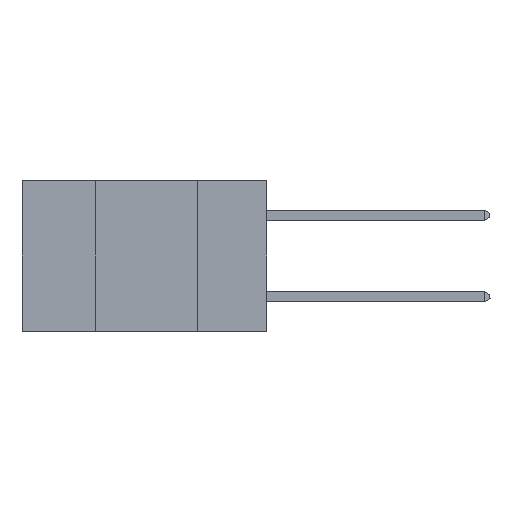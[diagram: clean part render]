
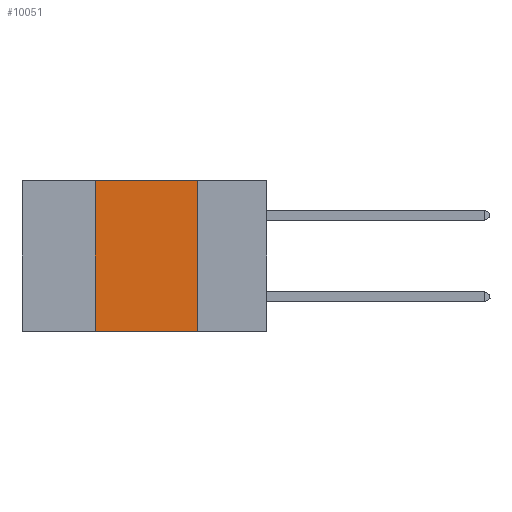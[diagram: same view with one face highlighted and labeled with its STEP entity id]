
A CAD part, left-side view. The second image highlights one B-rep face of the part: STEP entity #10051.
In plain terms, the highlighted planar face has unit normal (-1, 0, 0).
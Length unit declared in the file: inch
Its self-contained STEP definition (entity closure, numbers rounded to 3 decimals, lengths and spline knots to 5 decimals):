
#732 = CARTESIAN_POINT ( 'NONE',  ( 0., 0.17, 0. ) ) ;
#1130 = DIRECTION ( 'NONE',  ( 0., -1., 0. ) ) ;
#2882 = LINE ( 'NONE', #7137, #13762 ) ;
#3094 = ORIENTED_EDGE ( 'NONE', *, *, #14947, .F. ) ;
#3384 = EDGE_LOOP ( 'NONE', ( #3094, #11503, #5158, #14733 ) ) ;
#3385 = CARTESIAN_POINT ( 'NONE',  ( 0., 0.6, -0.37 ) ) ;
#3785 = VERTEX_POINT ( 'NONE', #13073 ) ;
#4126 = EDGE_CURVE ( 'NONE', #13854, #11864, #10080, .T. ) ;
#4193 = LINE ( 'NONE', #732, #5136 ) ;
#4670 = PLANE ( 'NONE',  #7033 ) ;
#5136 = VECTOR ( 'NONE', #6911, 39.37008 ) ;
#5158 = ORIENTED_EDGE ( 'NONE', *, *, #7703, .F. ) ;
#6596 = CARTESIAN_POINT ( 'NONE',  ( 0., 0.42, 0. ) ) ;
#6760 = VERTEX_POINT ( 'NONE', #15274 ) ;
#6911 = DIRECTION ( 'NONE',  ( 0., 0., -1. ) ) ;
#7033 = AXIS2_PLACEMENT_3D ( 'NONE', #14284, #12029, #15454 ) ;
#7137 = CARTESIAN_POINT ( 'NONE',  ( 0., 0.6, 0. ) ) ;
#7703 = EDGE_CURVE ( 'NONE', #13854, #3785, #9511, .T. ) ;
#8476 = FACE_OUTER_BOUND ( 'NONE', #3384, .T. ) ;
#9511 = LINE ( 'NONE', #6596, #12341 ) ;
#10051 = ADVANCED_FACE ( 'NONE', ( #8476 ), #4670, .F. ) ;
#10080 = LINE ( 'NONE', #3385, #15096 ) ;
#10211 = DIRECTION ( 'NONE',  ( 0., 0., 1. ) ) ;
#11503 = ORIENTED_EDGE ( 'NONE', *, *, #14409, .F. ) ;
#11864 = VERTEX_POINT ( 'NONE', #12557 ) ;
#12029 = DIRECTION ( 'NONE',  ( 1., 0., 0. ) ) ;
#12341 = VECTOR ( 'NONE', #10211, 39.37008 ) ;
#12557 = CARTESIAN_POINT ( 'NONE',  ( 0., 0.17, -0.37 ) ) ;
#13073 = CARTESIAN_POINT ( 'NONE',  ( 0., 0.42, 0. ) ) ;
#13762 = VECTOR ( 'NONE', #1130, 39.37008 ) ;
#13854 = VERTEX_POINT ( 'NONE', #14520 ) ;
#14015 = DIRECTION ( 'NONE',  ( 0., -1., 0. ) ) ;
#14284 = CARTESIAN_POINT ( 'NONE',  ( 0., 0.6, 0. ) ) ;
#14409 = EDGE_CURVE ( 'NONE', #3785, #6760, #2882, .T. ) ;
#14520 = CARTESIAN_POINT ( 'NONE',  ( 0., 0.42, -0.37 ) ) ;
#14733 = ORIENTED_EDGE ( 'NONE', *, *, #4126, .T. ) ;
#14947 = EDGE_CURVE ( 'NONE', #6760, #11864, #4193, .T. ) ;
#15096 = VECTOR ( 'NONE', #14015, 39.37008 ) ;
#15274 = CARTESIAN_POINT ( 'NONE',  ( 0., 0.17, 0. ) ) ;
#15454 = DIRECTION ( 'NONE',  ( 0., 0., -1. ) ) ;
